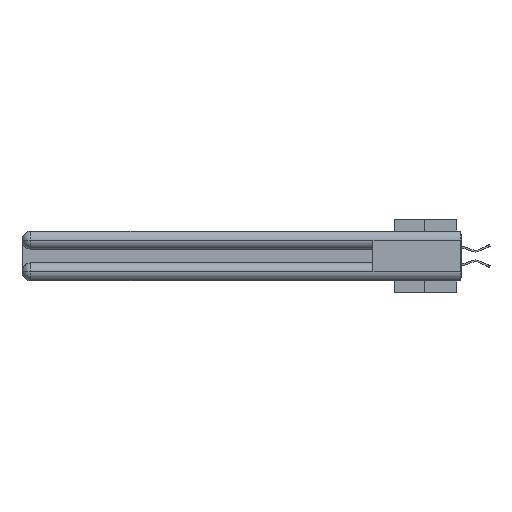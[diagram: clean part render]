
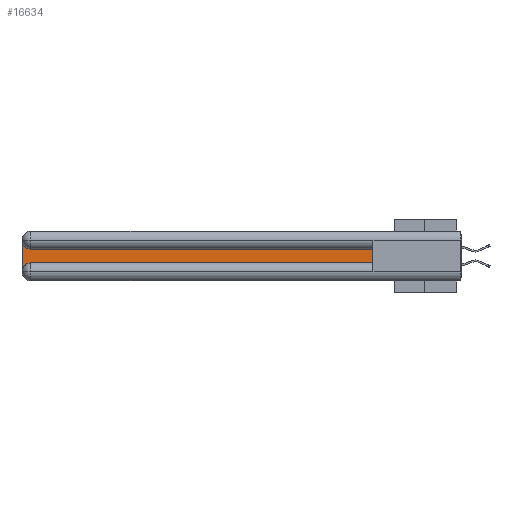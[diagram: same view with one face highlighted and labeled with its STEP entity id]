
A CAD part, left-side view. The second image highlights one B-rep face of the part: STEP entity #16634.
In plain terms, the highlighted planar face has unit normal (-1, 0, 0).
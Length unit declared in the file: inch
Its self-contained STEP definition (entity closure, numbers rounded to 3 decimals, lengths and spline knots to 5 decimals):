
#67 = CARTESIAN_POINT ( 'NONE',  ( 0.075, 3., -0.2775 ) ) ;
#142 = CARTESIAN_POINT ( 'NONE',  ( 0.075, 0.6, -0.2175 ) ) ;
#536 = EDGE_CURVE ( 'NONE', #39045, #1623, #39256, .T. ) ;
#736 = DIRECTION ( 'NONE',  ( 0., 0., -1. ) ) ;
#1623 = VERTEX_POINT ( 'NONE', #20422 ) ;
#1695 = ORIENTED_EDGE ( 'NONE', *, *, #19817, .T. ) ;
#2642 = DIRECTION ( 'NONE',  ( 0., 1., 0. ) ) ;
#2769 = ORIENTED_EDGE ( 'NONE', *, *, #3016, .T. ) ;
#3016 = EDGE_CURVE ( 'NONE', #36526, #31661, #3172, .T. ) ;
#3172 = CIRCLE ( 'NONE', #14706, 0.06 ) ;
#4864 = VECTOR ( 'NONE', #24543, 39.37008 ) ;
#5317 = CARTESIAN_POINT ( 'NONE',  ( 0.075, 0.6, -0.2175 ) ) ;
#5829 = CARTESIAN_POINT ( 'NONE',  ( 0.075, 0.6, -0.1225 ) ) ;
#6285 = VECTOR ( 'NONE', #32519, 39.37008 ) ;
#8987 = VERTEX_POINT ( 'NONE', #38697 ) ;
#9708 = PLANE ( 'NONE',  #38599 ) ;
#9766 = AXIS2_PLACEMENT_3D ( 'NONE', #30734, #33793, #21666 ) ;
#9914 = DIRECTION ( 'NONE',  ( 1., 0., 0. ) ) ;
#9938 = CARTESIAN_POINT ( 'NONE',  ( 0.075, 0.6, -0.2175 ) ) ;
#11571 = LINE ( 'NONE', #142, #4864 ) ;
#12058 = CARTESIAN_POINT ( 'NONE',  ( 0.075, 3., -0.2175 ) ) ;
#14706 = AXIS2_PLACEMENT_3D ( 'NONE', #25108, #9914, #31361 ) ;
#15978 = EDGE_LOOP ( 'NONE', ( #28925, #32336, #34610, #2769, #33658, #1695 ) ) ;
#16634 = ADVANCED_FACE ( 'NONE', ( #23157 ), #9708, .F. ) ;
#17383 = CARTESIAN_POINT ( 'NONE',  ( 0.075, 2.94, -0.1225 ) ) ;
#18603 = DIRECTION ( 'NONE',  ( 0., 0., -1. ) ) ;
#19312 = LINE ( 'NONE', #5829, #22207 ) ;
#19817 = EDGE_CURVE ( 'NONE', #25935, #8987, #11571, .T. ) ;
#19872 = EDGE_CURVE ( 'NONE', #1623, #36526, #36990, .T. ) ;
#20422 = CARTESIAN_POINT ( 'NONE',  ( 0.075, 3., -0.0625 ) ) ;
#21666 = DIRECTION ( 'NONE',  ( 0., 0., -1. ) ) ;
#22207 = VECTOR ( 'NONE', #2642, 39.37008 ) ;
#23157 = FACE_OUTER_BOUND ( 'NONE', #15978, .T. ) ;
#24543 = DIRECTION ( 'NONE',  ( 0., 0., 1. ) ) ;
#25108 = CARTESIAN_POINT ( 'NONE',  ( 0.075, 2.94, -0.2775 ) ) ;
#25935 = VERTEX_POINT ( 'NONE', #9938 ) ;
#27865 = VECTOR ( 'NONE', #18603, 39.37008 ) ;
#28535 = CARTESIAN_POINT ( 'NONE',  ( 0.075, 2.94, -0.2175 ) ) ;
#28925 = ORIENTED_EDGE ( 'NONE', *, *, #29776, .T. ) ;
#29776 = EDGE_CURVE ( 'NONE', #8987, #39045, #19312, .T. ) ;
#30734 = CARTESIAN_POINT ( 'NONE',  ( 0.075, 2.94, -0.0625 ) ) ;
#31148 = CARTESIAN_POINT ( 'NONE',  ( 0.075, 3., -0.1225 ) ) ;
#31361 = DIRECTION ( 'NONE',  ( 0., 0., -1. ) ) ;
#31661 = VERTEX_POINT ( 'NONE', #28535 ) ;
#32336 = ORIENTED_EDGE ( 'NONE', *, *, #536, .T. ) ;
#32519 = DIRECTION ( 'NONE',  ( 0., -1., 0. ) ) ;
#33658 = ORIENTED_EDGE ( 'NONE', *, *, #36052, .T. ) ;
#33793 = DIRECTION ( 'NONE',  ( 1., 0., 0. ) ) ;
#34205 = DIRECTION ( 'NONE',  ( 1., 0., 0. ) ) ;
#34610 = ORIENTED_EDGE ( 'NONE', *, *, #19872, .T. ) ;
#35053 = LINE ( 'NONE', #5317, #6285 ) ;
#36052 = EDGE_CURVE ( 'NONE', #31661, #25935, #35053, .T. ) ;
#36526 = VERTEX_POINT ( 'NONE', #67 ) ;
#36990 = LINE ( 'NONE', #12058, #27865 ) ;
#38599 = AXIS2_PLACEMENT_3D ( 'NONE', #31148, #34205, #736 ) ;
#38697 = CARTESIAN_POINT ( 'NONE',  ( 0.075, 0.6, -0.1225 ) ) ;
#39045 = VERTEX_POINT ( 'NONE', #17383 ) ;
#39256 = CIRCLE ( 'NONE', #9766, 0.06 ) ;
